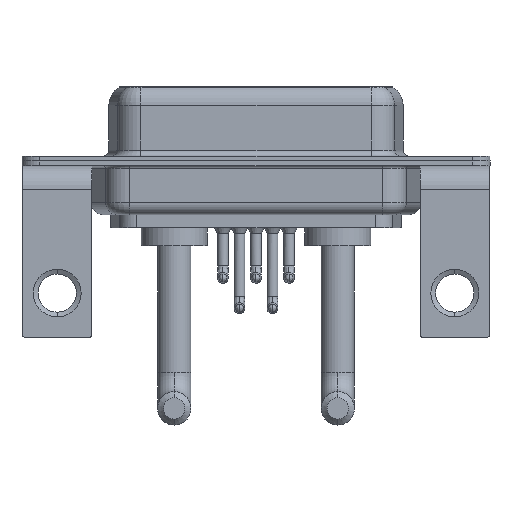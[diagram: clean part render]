
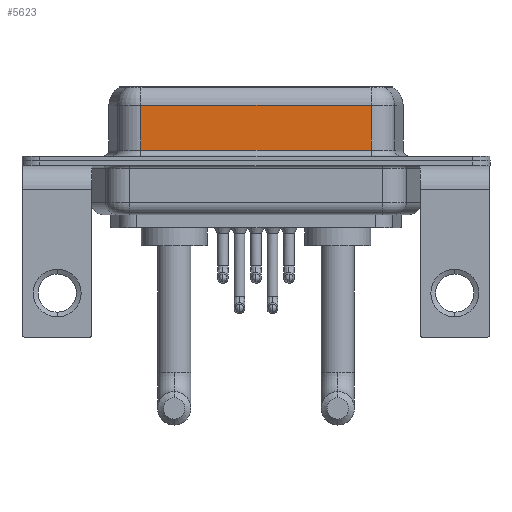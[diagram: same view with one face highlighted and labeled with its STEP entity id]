
A CAD part, front view. The second image highlights one B-rep face of the part: STEP entity #5623.
In plain terms, the highlighted planar face has unit normal (0, -1, 0).
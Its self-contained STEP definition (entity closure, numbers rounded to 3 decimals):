
#1372 = EDGE_LOOP ( 'NONE', ( #17496, #5988, #14158, #10473 ) ) ;
#2868 = VECTOR ( 'NONE', #10371, 1000. ) ;
#4752 = LINE ( 'NONE', #11792, #14494 ) ;
#5623 = ADVANCED_FACE ( 'NONE', ( #6052 ), #12931, .F. ) ;
#5988 = ORIENTED_EDGE ( 'NONE', *, *, #12262, .T. ) ;
#6052 = FACE_OUTER_BOUND ( 'NONE', #1372, .T. ) ;
#6299 = DIRECTION ( 'NONE',  ( -1., 0., 0. ) ) ;
#7891 = CARTESIAN_POINT ( 'NONE',  ( 26.287, -3.95, 4.65 ) ) ;
#8074 = CARTESIAN_POINT ( 'NONE',  ( 7.013, -3.95, 0.9 ) ) ;
#8564 = EDGE_CURVE ( 'NONE', #13254, #15618, #4752, .T. ) ;
#8739 = LINE ( 'NONE', #11606, #9638 ) ;
#8746 = AXIS2_PLACEMENT_3D ( 'NONE', #12844, #11512, #12666 ) ;
#8905 = EDGE_CURVE ( 'NONE', #10861, #15618, #8739, .T. ) ;
#8984 = LINE ( 'NONE', #13012, #15478 ) ;
#9638 = VECTOR ( 'NONE', #17146, 1000. ) ;
#9747 = VERTEX_POINT ( 'NONE', #13072 ) ;
#10371 = DIRECTION ( 'NONE',  ( 0., 0., -1. ) ) ;
#10473 = ORIENTED_EDGE ( 'NONE', *, *, #8905, .T. ) ;
#10861 = VERTEX_POINT ( 'NONE', #8074 ) ;
#11512 = DIRECTION ( 'NONE',  ( 0., 1., 0. ) ) ;
#11606 = CARTESIAN_POINT ( 'NONE',  ( 26.287, -3.95, 0.9 ) ) ;
#11792 = CARTESIAN_POINT ( 'NONE',  ( 26.287, -3.95, 6.4 ) ) ;
#11873 = DIRECTION ( 'NONE',  ( 0., 0., -1. ) ) ;
#12262 = EDGE_CURVE ( 'NONE', #13254, #9747, #8984, .T. ) ;
#12666 = DIRECTION ( 'NONE',  ( 0., 0., 1. ) ) ;
#12844 = CARTESIAN_POINT ( 'NONE',  ( 26.287, -3.95, 6.4 ) ) ;
#12931 = PLANE ( 'NONE',  #8746 ) ;
#13012 = CARTESIAN_POINT ( 'NONE',  ( 26.287, -3.95, 4.65 ) ) ;
#13072 = CARTESIAN_POINT ( 'NONE',  ( 7.013, -3.95, 4.65 ) ) ;
#13254 = VERTEX_POINT ( 'NONE', #7891 ) ;
#13921 = EDGE_CURVE ( 'NONE', #9747, #10861, #16997, .T. ) ;
#14158 = ORIENTED_EDGE ( 'NONE', *, *, #13921, .T. ) ;
#14461 = CARTESIAN_POINT ( 'NONE',  ( 7.013, -3.95, 6.4 ) ) ;
#14494 = VECTOR ( 'NONE', #11873, 1000. ) ;
#15478 = VECTOR ( 'NONE', #6299, 1000. ) ;
#15618 = VERTEX_POINT ( 'NONE', #15979 ) ;
#15979 = CARTESIAN_POINT ( 'NONE',  ( 26.287, -3.95, 0.9 ) ) ;
#16997 = LINE ( 'NONE', #14461, #2868 ) ;
#17146 = DIRECTION ( 'NONE',  ( 1., 0., 0. ) ) ;
#17496 = ORIENTED_EDGE ( 'NONE', *, *, #8564, .F. ) ;
